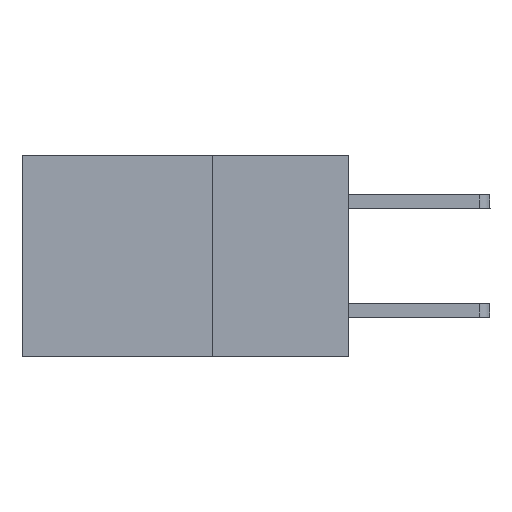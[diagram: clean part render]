
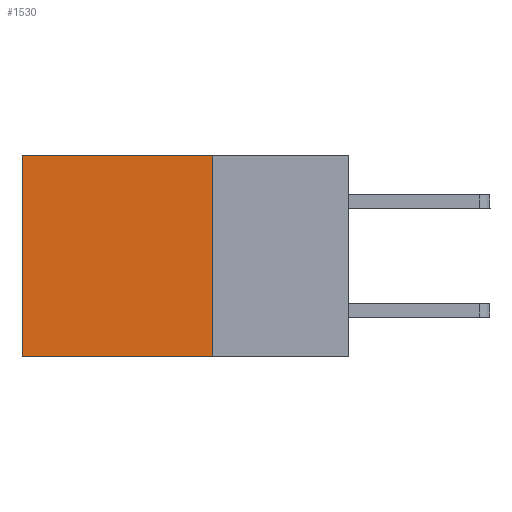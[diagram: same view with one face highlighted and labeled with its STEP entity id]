
A CAD part, left-side view. The second image highlights one B-rep face of the part: STEP entity #1530.
In plain terms, the highlighted planar face has unit normal (-1, 0, 0).
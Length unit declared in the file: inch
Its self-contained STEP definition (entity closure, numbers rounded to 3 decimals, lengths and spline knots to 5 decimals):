
#190 = DIRECTION ( 'NONE',  ( 0., 1., 0. ) ) ;
#357 = VECTOR ( 'NONE', #4011, 39.37008 ) ;
#359 = EDGE_LOOP ( 'NONE', ( #3708, #5727, #8824, #1116 ) ) ;
#571 = EDGE_CURVE ( 'NONE', #8297, #1248, #8877, .T. ) ;
#693 = CARTESIAN_POINT ( 'NONE',  ( 0.2615, 0.25, -0.37 ) ) ;
#967 = CARTESIAN_POINT ( 'NONE',  ( 0.2615, 0.6, -0.37 ) ) ;
#995 = CARTESIAN_POINT ( 'NONE',  ( 0.2615, 0.6, 0. ) ) ;
#1116 = ORIENTED_EDGE ( 'NONE', *, *, #6923, .T. ) ;
#1216 = CARTESIAN_POINT ( 'NONE',  ( 0.2615, 0.25, -0.37 ) ) ;
#1248 = VERTEX_POINT ( 'NONE', #967 ) ;
#1530 = ADVANCED_FACE ( 'NONE', ( #4050 ), #5546, .F. ) ;
#2054 = VECTOR ( 'NONE', #190, 39.37008 ) ;
#2055 = LINE ( 'NONE', #3346, #357 ) ;
#2956 = AXIS2_PLACEMENT_3D ( 'NONE', #5502, #4650, #8800 ) ;
#3022 = CARTESIAN_POINT ( 'NONE',  ( 0.2615, 0.25, 0. ) ) ;
#3147 = EDGE_CURVE ( 'NONE', #5969, #8297, #7470, .T. ) ;
#3346 = CARTESIAN_POINT ( 'NONE',  ( 0.2615, 0.6, -0.37 ) ) ;
#3708 = ORIENTED_EDGE ( 'NONE', *, *, #5494, .T. ) ;
#3989 = VECTOR ( 'NONE', #7514, 39.37008 ) ;
#4011 = DIRECTION ( 'NONE',  ( 0., 0., -1. ) ) ;
#4050 = FACE_OUTER_BOUND ( 'NONE', #359, .T. ) ;
#4332 = LINE ( 'NONE', #3022, #8810 ) ;
#4650 = DIRECTION ( 'NONE',  ( 1., 0., 0. ) ) ;
#5286 = VERTEX_POINT ( 'NONE', #995 ) ;
#5494 = EDGE_CURVE ( 'NONE', #5286, #1248, #2055, .T. ) ;
#5502 = CARTESIAN_POINT ( 'NONE',  ( 0.2615, 0.25, -0.37 ) ) ;
#5542 = CARTESIAN_POINT ( 'NONE',  ( 0.2615, 0.25, -0.37 ) ) ;
#5546 = PLANE ( 'NONE',  #2956 ) ;
#5727 = ORIENTED_EDGE ( 'NONE', *, *, #571, .F. ) ;
#5969 = VERTEX_POINT ( 'NONE', #8232 ) ;
#6923 = EDGE_CURVE ( 'NONE', #5969, #5286, #4332, .T. ) ;
#7199 = DIRECTION ( 'NONE',  ( 0., 1., 0. ) ) ;
#7470 = LINE ( 'NONE', #1216, #3989 ) ;
#7514 = DIRECTION ( 'NONE',  ( 0., 0., -1. ) ) ;
#8232 = CARTESIAN_POINT ( 'NONE',  ( 0.2615, 0.25, 0. ) ) ;
#8297 = VERTEX_POINT ( 'NONE', #693 ) ;
#8800 = DIRECTION ( 'NONE',  ( 0., 0., -1. ) ) ;
#8810 = VECTOR ( 'NONE', #7199, 39.37008 ) ;
#8824 = ORIENTED_EDGE ( 'NONE', *, *, #3147, .F. ) ;
#8877 = LINE ( 'NONE', #5542, #2054 ) ;
